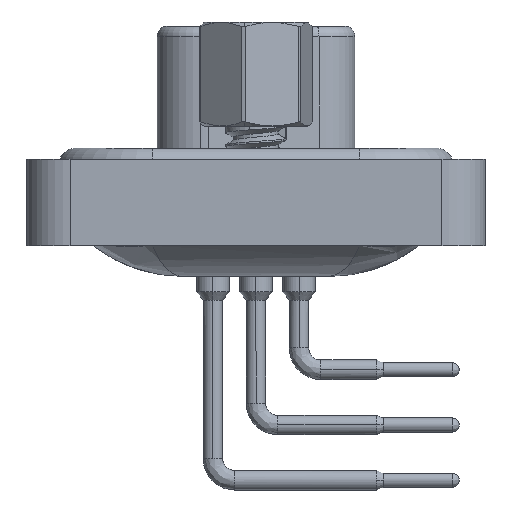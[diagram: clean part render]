
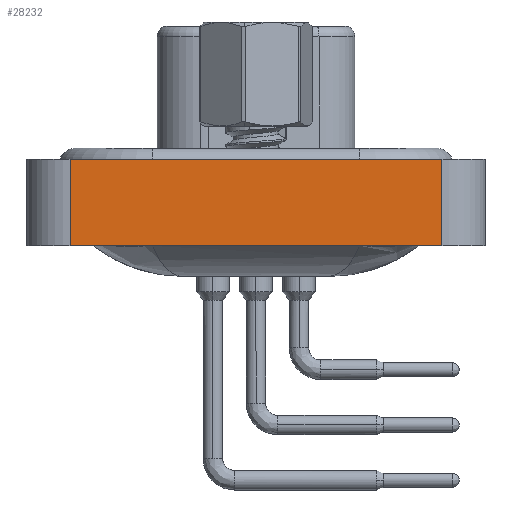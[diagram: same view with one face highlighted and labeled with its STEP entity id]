
A CAD part, left-side view. The second image highlights one B-rep face of the part: STEP entity #28232.
In plain terms, the highlighted planar face has unit normal (-1, 0, 0).
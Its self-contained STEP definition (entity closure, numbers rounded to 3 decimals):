
#2061 = CARTESIAN_POINT ( 'NONE',  ( -7.285, -8.55, 0.4 ) ) ;
#2231 = CARTESIAN_POINT ( 'NONE',  ( -7.285, 8.55, -3.6 ) ) ;
#2556 = CARTESIAN_POINT ( 'NONE',  ( -7.285, -8.55, 0.4 ) ) ;
#3217 = EDGE_CURVE ( 'NONE', #9084, #25048, #5183, .T. ) ;
#3751 = CARTESIAN_POINT ( 'NONE',  ( -7.285, -8.55, -3.6 ) ) ;
#5183 = LINE ( 'NONE', #22057, #10424 ) ;
#7417 = DIRECTION ( 'NONE',  ( -1., 0., 0. ) ) ;
#8097 = CARTESIAN_POINT ( 'NONE',  ( -7.285, 8.55, 0.4 ) ) ;
#8428 = EDGE_CURVE ( 'NONE', #32163, #9084, #19932, .T. ) ;
#9084 = VERTEX_POINT ( 'NONE', #29521 ) ;
#9813 = EDGE_LOOP ( 'NONE', ( #27328, #26383, #28351, #13535 ) ) ;
#10114 = PLANE ( 'NONE',  #23296 ) ;
#10301 = EDGE_CURVE ( 'NONE', #11344, #25048, #27140, .T. ) ;
#10424 = VECTOR ( 'NONE', #29760, 1000. ) ;
#11344 = VERTEX_POINT ( 'NONE', #8097 ) ;
#13199 = DIRECTION ( 'NONE',  ( 0., 0., 1. ) ) ;
#13535 = ORIENTED_EDGE ( 'NONE', *, *, #8428, .T. ) ;
#18946 = LINE ( 'NONE', #2231, #26122 ) ;
#19747 = CARTESIAN_POINT ( 'NONE',  ( -7.285, 8.55, -3.6 ) ) ;
#19932 = LINE ( 'NONE', #3751, #21711 ) ;
#21079 = DIRECTION ( 'NONE',  ( 0., 0., 1. ) ) ;
#21711 = VECTOR ( 'NONE', #22614, 1000. ) ;
#22057 = CARTESIAN_POINT ( 'NONE',  ( -7.285, -8.55, -3.6 ) ) ;
#22614 = DIRECTION ( 'NONE',  ( 0., -1., 0. ) ) ;
#23120 = VECTOR ( 'NONE', #30006, 1000. ) ;
#23296 = AXIS2_PLACEMENT_3D ( 'NONE', #24450, #7417, #21079 ) ;
#24450 = CARTESIAN_POINT ( 'NONE',  ( -7.285, -8.55, -3.6 ) ) ;
#25048 = VERTEX_POINT ( 'NONE', #2061 ) ;
#26122 = VECTOR ( 'NONE', #13199, 1000. ) ;
#26383 = ORIENTED_EDGE ( 'NONE', *, *, #10301, .F. ) ;
#27140 = LINE ( 'NONE', #2556, #23120 ) ;
#27328 = ORIENTED_EDGE ( 'NONE', *, *, #3217, .T. ) ;
#27768 = EDGE_CURVE ( 'NONE', #32163, #11344, #18946, .T. ) ;
#28232 = ADVANCED_FACE ( 'NONE', ( #29647 ), #10114, .T. ) ;
#28351 = ORIENTED_EDGE ( 'NONE', *, *, #27768, .F. ) ;
#29521 = CARTESIAN_POINT ( 'NONE',  ( -7.285, -8.55, -3.6 ) ) ;
#29647 = FACE_OUTER_BOUND ( 'NONE', #9813, .T. ) ;
#29760 = DIRECTION ( 'NONE',  ( 0., 0., 1. ) ) ;
#30006 = DIRECTION ( 'NONE',  ( 0., -1., 0. ) ) ;
#32163 = VERTEX_POINT ( 'NONE', #19747 ) ;
